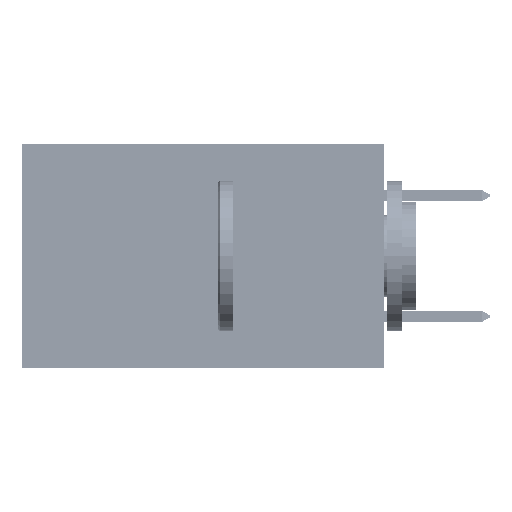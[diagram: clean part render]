
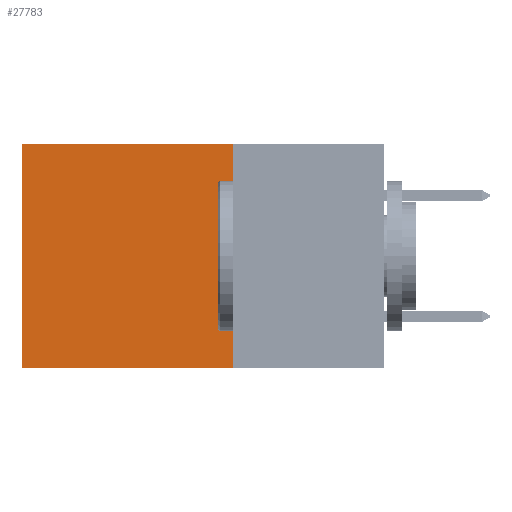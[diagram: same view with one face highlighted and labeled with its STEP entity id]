
A CAD part, left-side view. The second image highlights one B-rep face of the part: STEP entity #27783.
In plain terms, the highlighted planar face has unit normal (-1, 0, 0).
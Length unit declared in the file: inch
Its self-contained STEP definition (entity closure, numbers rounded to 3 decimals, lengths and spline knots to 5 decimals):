
#464 = VECTOR ( 'NONE', #44409, 39.37008 ) ;
#1199 = LINE ( 'NONE', #34565, #41075 ) ;
#2085 = CARTESIAN_POINT ( 'NONE',  ( 0.2875, 0.6, 0. ) ) ;
#2930 = CARTESIAN_POINT ( 'NONE',  ( 0.2875, 0.25, 0. ) ) ;
#3428 = DIRECTION ( 'NONE',  ( 0., 1., 0. ) ) ;
#3488 = CARTESIAN_POINT ( 'NONE',  ( 0.2875, 0.6, -0.37 ) ) ;
#4768 = VERTEX_POINT ( 'NONE', #2085 ) ;
#8259 = DIRECTION ( 'NONE',  ( 1., 0., 0. ) ) ;
#8910 = DIRECTION ( 'NONE',  ( 0., 0., -1. ) ) ;
#12362 = PLANE ( 'NONE',  #13020 ) ;
#13020 = AXIS2_PLACEMENT_3D ( 'NONE', #24423, #8259, #20097 ) ;
#13967 = DIRECTION ( 'NONE',  ( 0., 0., -1. ) ) ;
#16036 = CARTESIAN_POINT ( 'NONE',  ( 0.2875, 0.25, -0.37 ) ) ;
#18230 = EDGE_CURVE ( 'NONE', #32966, #45025, #46443, .T. ) ;
#18844 = ORIENTED_EDGE ( 'NONE', *, *, #40905, .T. ) ;
#20097 = DIRECTION ( 'NONE',  ( 0., 0., -1. ) ) ;
#21506 = EDGE_LOOP ( 'NONE', ( #37282, #42447, #25617, #18844 ) ) ;
#24423 = CARTESIAN_POINT ( 'NONE',  ( 0.2875, 0.25, 0. ) ) ;
#25617 = ORIENTED_EDGE ( 'NONE', *, *, #51647, .F. ) ;
#27783 = ADVANCED_FACE ( 'NONE', ( #50677 ), #12362, .F. ) ;
#29397 = LINE ( 'NONE', #2930, #464 ) ;
#32966 = VERTEX_POINT ( 'NONE', #16036 ) ;
#34565 = CARTESIAN_POINT ( 'NONE',  ( 0.2875, 0.25, 0. ) ) ;
#37282 = ORIENTED_EDGE ( 'NONE', *, *, #43301, .T. ) ;
#37363 = CARTESIAN_POINT ( 'NONE',  ( 0.2875, 0.25, 0. ) ) ;
#38086 = CARTESIAN_POINT ( 'NONE',  ( 0.2875, 0.6, 0. ) ) ;
#40905 = EDGE_CURVE ( 'NONE', #49311, #4768, #29397, .T. ) ;
#41075 = VECTOR ( 'NONE', #13967, 39.37008 ) ;
#42447 = ORIENTED_EDGE ( 'NONE', *, *, #18230, .F. ) ;
#43301 = EDGE_CURVE ( 'NONE', #4768, #45025, #46435, .T. ) ;
#44211 = CARTESIAN_POINT ( 'NONE',  ( 0.2875, 0.25, -0.37 ) ) ;
#44409 = DIRECTION ( 'NONE',  ( 0., 1., 0. ) ) ;
#45025 = VERTEX_POINT ( 'NONE', #3488 ) ;
#45157 = VECTOR ( 'NONE', #3428, 39.37008 ) ;
#46435 = LINE ( 'NONE', #38086, #50320 ) ;
#46443 = LINE ( 'NONE', #44211, #45157 ) ;
#49311 = VERTEX_POINT ( 'NONE', #37363 ) ;
#50320 = VECTOR ( 'NONE', #8910, 39.37008 ) ;
#50677 = FACE_OUTER_BOUND ( 'NONE', #21506, .T. ) ;
#51647 = EDGE_CURVE ( 'NONE', #49311, #32966, #1199, .T. ) ;
